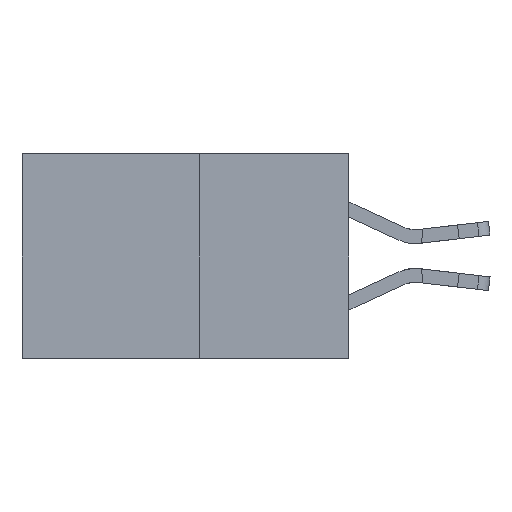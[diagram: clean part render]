
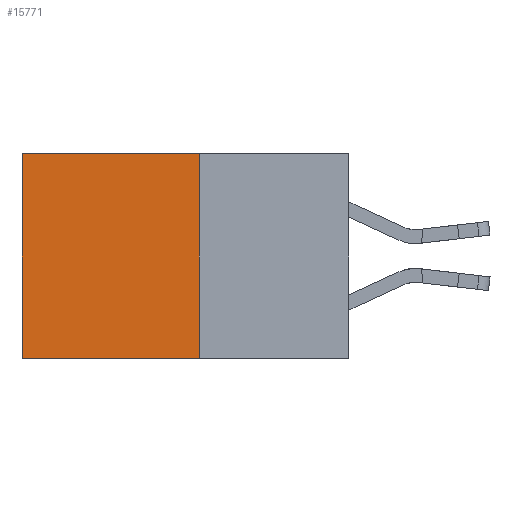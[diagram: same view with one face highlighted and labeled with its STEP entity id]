
A CAD part, left-side view. The second image highlights one B-rep face of the part: STEP entity #15771.
In plain terms, the highlighted planar face has unit normal (-1, 0, 0).
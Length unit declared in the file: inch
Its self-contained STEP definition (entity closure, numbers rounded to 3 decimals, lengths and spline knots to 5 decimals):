
#276 = CARTESIAN_POINT ( 'NONE',  ( 0.277, 0.27, -0.37 ) ) ;
#1113 = VERTEX_POINT ( 'NONE', #1840 ) ;
#1840 = CARTESIAN_POINT ( 'NONE',  ( 0.277, 0.27, 0. ) ) ;
#1877 = VERTEX_POINT ( 'NONE', #276 ) ;
#4216 = EDGE_CURVE ( 'NONE', #1877, #23518, #26812, .T. ) ;
#4339 = VECTOR ( 'NONE', #28636, 39.37008 ) ;
#4574 = ORIENTED_EDGE ( 'NONE', *, *, #18976, .T. ) ;
#4894 = LINE ( 'NONE', #14853, #16199 ) ;
#5049 = LINE ( 'NONE', #6502, #4339 ) ;
#5220 = ORIENTED_EDGE ( 'NONE', *, *, #11634, .F. ) ;
#6502 = CARTESIAN_POINT ( 'NONE',  ( 0.277, 0.27, 0. ) ) ;
#7192 = FACE_OUTER_BOUND ( 'NONE', #7331, .T. ) ;
#7331 = EDGE_LOOP ( 'NONE', ( #4574, #21189, #5220, #13433 ) ) ;
#8471 = DIRECTION ( 'NONE',  ( 1., 0., 0. ) ) ;
#10253 = CARTESIAN_POINT ( 'NONE',  ( 0.277, 0.59, 0. ) ) ;
#11634 = EDGE_CURVE ( 'NONE', #1113, #1877, #4894, .T. ) ;
#11758 = CARTESIAN_POINT ( 'NONE',  ( 0.277, 0.59, -0.37 ) ) ;
#12685 = DIRECTION ( 'NONE',  ( 0., 0., -1. ) ) ;
#12705 = VECTOR ( 'NONE', #25036, 39.37008 ) ;
#13433 = ORIENTED_EDGE ( 'NONE', *, *, #15869, .T. ) ;
#14853 = CARTESIAN_POINT ( 'NONE',  ( 0.277, 0.27, -0.37 ) ) ;
#15635 = VERTEX_POINT ( 'NONE', #10253 ) ;
#15771 = ADVANCED_FACE ( 'NONE', ( #7192 ), #21912, .F. ) ;
#15869 = EDGE_CURVE ( 'NONE', #1113, #15635, #5049, .T. ) ;
#16199 = VECTOR ( 'NONE', #12685, 39.37008 ) ;
#17452 = CARTESIAN_POINT ( 'NONE',  ( 0.277, 0.27, -0.37 ) ) ;
#18109 = CARTESIAN_POINT ( 'NONE',  ( 0.277, 0.59, -0.37 ) ) ;
#18460 = CARTESIAN_POINT ( 'NONE',  ( 0.277, 0.27, -0.37 ) ) ;
#18976 = EDGE_CURVE ( 'NONE', #15635, #23518, #24517, .T. ) ;
#21189 = ORIENTED_EDGE ( 'NONE', *, *, #4216, .F. ) ;
#21788 = VECTOR ( 'NONE', #26657, 39.37008 ) ;
#21912 = PLANE ( 'NONE',  #25135 ) ;
#23518 = VERTEX_POINT ( 'NONE', #18109 ) ;
#24098 = DIRECTION ( 'NONE',  ( 0., 0., -1. ) ) ;
#24517 = LINE ( 'NONE', #11758, #12705 ) ;
#25036 = DIRECTION ( 'NONE',  ( 0., 0., -1. ) ) ;
#25135 = AXIS2_PLACEMENT_3D ( 'NONE', #17452, #8471, #24098 ) ;
#26657 = DIRECTION ( 'NONE',  ( 0., 1., 0. ) ) ;
#26812 = LINE ( 'NONE', #18460, #21788 ) ;
#28636 = DIRECTION ( 'NONE',  ( 0., 1., 0. ) ) ;
